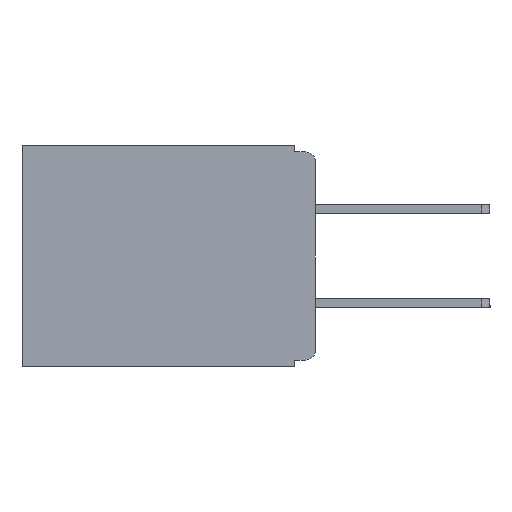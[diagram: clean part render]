
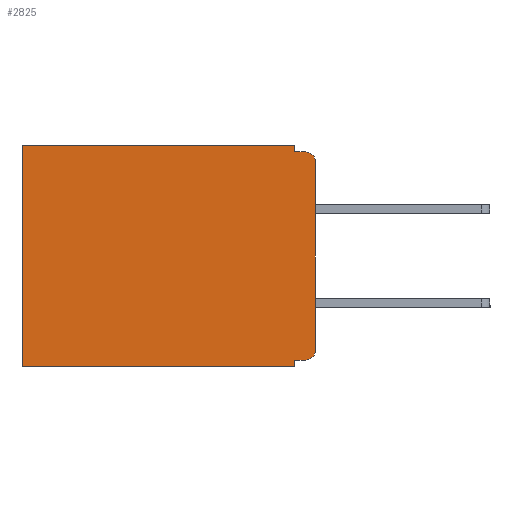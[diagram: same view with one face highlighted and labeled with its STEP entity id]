
A CAD part, left-side view. The second image highlights one B-rep face of the part: STEP entity #2825.
In plain terms, the highlighted planar face has unit normal (-1, 0, 0).
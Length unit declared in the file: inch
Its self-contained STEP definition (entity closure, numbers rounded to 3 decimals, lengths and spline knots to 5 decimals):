
#13 = ORIENTED_EDGE ( 'NONE', *, *, #7940, .T. ) ;
#251 = ORIENTED_EDGE ( 'NONE', *, *, #16608, .T. ) ;
#423 = EDGE_CURVE ( 'NONE', #15945, #10804, #10420, .T. ) ;
#532 = ORIENTED_EDGE ( 'NONE', *, *, #8888, .F. ) ;
#535 = DIRECTION ( 'NONE',  ( 0., 1., 0. ) ) ;
#1096 = ORIENTED_EDGE ( 'NONE', *, *, #5507, .F. ) ;
#1252 = ORIENTED_EDGE ( 'NONE', *, *, #423, .T. ) ;
#1308 = EDGE_CURVE ( 'NONE', #12455, #4254, #18576, .T. ) ;
#1642 = LINE ( 'NONE', #11935, #13203 ) ;
#1795 = CARTESIAN_POINT ( 'NONE',  ( 0.3, 0.031, 0. ) ) ;
#2652 = DIRECTION ( 'NONE',  ( -1., 0., 0. ) ) ;
#2656 = VERTEX_POINT ( 'NONE', #4014 ) ;
#2825 = ADVANCED_FACE ( 'NONE', ( #13002 ), #16851, .F. ) ;
#2857 = CARTESIAN_POINT ( 'NONE',  ( 0.3, 0., -0.33 ) ) ;
#2863 = DIRECTION ( 'NONE',  ( 0., 0., -1. ) ) ;
#3182 = EDGE_CURVE ( 'NONE', #6920, #4254, #11863, .T. ) ;
#3349 = VECTOR ( 'NONE', #5999, 39.37008 ) ;
#3707 = CARTESIAN_POINT ( 'NONE',  ( 0.3, 0.437, -0.33 ) ) ;
#4014 = CARTESIAN_POINT ( 'NONE',  ( 0.3, 0.031, -0.01 ) ) ;
#4216 = CIRCLE ( 'NONE', #11251, 0.015 ) ;
#4254 = VERTEX_POINT ( 'NONE', #3707 ) ;
#4491 = LINE ( 'NONE', #16780, #12026 ) ;
#5507 = EDGE_CURVE ( 'NONE', #2656, #15579, #18805, .T. ) ;
#5581 = ORIENTED_EDGE ( 'NONE', *, *, #7904, .F. ) ;
#5868 = ORIENTED_EDGE ( 'NONE', *, *, #1308, .F. ) ;
#5924 = ORIENTED_EDGE ( 'NONE', *, *, #3182, .T. ) ;
#5999 = DIRECTION ( 'NONE',  ( 0., 0., -1. ) ) ;
#6069 = VERTEX_POINT ( 'NONE', #14376 ) ;
#6560 = DIRECTION ( 'NONE',  ( 0., -1., 0. ) ) ;
#6920 = VERTEX_POINT ( 'NONE', #17033 ) ;
#7224 = CARTESIAN_POINT ( 'NONE',  ( 0.3, 0., -0.01 ) ) ;
#7368 = ORIENTED_EDGE ( 'NONE', *, *, #13841, .F. ) ;
#7381 = DIRECTION ( 'NONE',  ( 0., 0., -1. ) ) ;
#7577 = VECTOR ( 'NONE', #6560, 39.37008 ) ;
#7847 = ORIENTED_EDGE ( 'NONE', *, *, #17361, .F. ) ;
#7904 = EDGE_CURVE ( 'NONE', #6069, #12455, #16985, .T. ) ;
#7940 = EDGE_CURVE ( 'NONE', #9602, #15579, #4216, .T. ) ;
#7973 = CARTESIAN_POINT ( 'NONE',  ( 0.3, 0., -0.33 ) ) ;
#8722 = DIRECTION ( 'NONE',  ( 0., 1., 0. ) ) ;
#8888 = EDGE_CURVE ( 'NONE', #15779, #2656, #19001, .T. ) ;
#9524 = DIRECTION ( 'NONE',  ( 0., 1., 0. ) ) ;
#9602 = VERTEX_POINT ( 'NONE', #13423 ) ;
#10281 = AXIS2_PLACEMENT_3D ( 'NONE', #18841, #2652, #2863 ) ;
#10314 = DIRECTION ( 'NONE',  ( 0., 0., -1. ) ) ;
#10359 = VECTOR ( 'NONE', #7381, 39.37008 ) ;
#10362 = DIRECTION ( 'NONE',  ( -1., 0., 0. ) ) ;
#10381 = CARTESIAN_POINT ( 'NONE',  ( 0.3, 0.015, -0.025 ) ) ;
#10420 = CIRCLE ( 'NONE', #10281, 0.015 ) ;
#10777 = DIRECTION ( 'NONE',  ( 0., 0., -1. ) ) ;
#10804 = VERTEX_POINT ( 'NONE', #16427 ) ;
#10861 = CARTESIAN_POINT ( 'NONE',  ( 0.3, 0.031, -0.33 ) ) ;
#11251 = AXIS2_PLACEMENT_3D ( 'NONE', #10381, #10362, #10314 ) ;
#11353 = CARTESIAN_POINT ( 'NONE',  ( 0.3, 0.015, -0.32 ) ) ;
#11863 = LINE ( 'NONE', #16821, #3349 ) ;
#11935 = CARTESIAN_POINT ( 'NONE',  ( 0.3, 0., -0.33 ) ) ;
#12026 = VECTOR ( 'NONE', #9524, 39.37008 ) ;
#12348 = LINE ( 'NONE', #18947, #19133 ) ;
#12455 = VERTEX_POINT ( 'NONE', #17919 ) ;
#13002 = FACE_OUTER_BOUND ( 'NONE', #13007, .T. ) ;
#13007 = EDGE_LOOP ( 'NONE', ( #7847, #13, #1096, #532, #251, #5924, #5868, #5581, #7368, #1252 ) ) ;
#13203 = VECTOR ( 'NONE', #13376, 39.37008 ) ;
#13376 = DIRECTION ( 'NONE',  ( 0., 0., -1. ) ) ;
#13423 = CARTESIAN_POINT ( 'NONE',  ( 0.3, 0., -0.025 ) ) ;
#13841 = EDGE_CURVE ( 'NONE', #15945, #6069, #4491, .T. ) ;
#14198 = AXIS2_PLACEMENT_3D ( 'NONE', #7973, #18688, #17633 ) ;
#14232 = VECTOR ( 'NONE', #535, 39.37008 ) ;
#14376 = CARTESIAN_POINT ( 'NONE',  ( 0.3, 0.031, -0.32 ) ) ;
#15579 = VERTEX_POINT ( 'NONE', #16243 ) ;
#15779 = VERTEX_POINT ( 'NONE', #1795 ) ;
#15945 = VERTEX_POINT ( 'NONE', #11353 ) ;
#16066 = VECTOR ( 'NONE', #10777, 39.37008 ) ;
#16243 = CARTESIAN_POINT ( 'NONE',  ( 0.3, 0.015, -0.01 ) ) ;
#16427 = CARTESIAN_POINT ( 'NONE',  ( 0.3, 0., -0.305 ) ) ;
#16608 = EDGE_CURVE ( 'NONE', #15779, #6920, #12348, .T. ) ;
#16780 = CARTESIAN_POINT ( 'NONE',  ( 0.3, 0., -0.32 ) ) ;
#16821 = CARTESIAN_POINT ( 'NONE',  ( 0.3, 0.437, -0.33 ) ) ;
#16851 = PLANE ( 'NONE',  #14198 ) ;
#16985 = LINE ( 'NONE', #10861, #16066 ) ;
#17033 = CARTESIAN_POINT ( 'NONE',  ( 0.3, 0.437, 0. ) ) ;
#17361 = EDGE_CURVE ( 'NONE', #9602, #10804, #1642, .T. ) ;
#17567 = CARTESIAN_POINT ( 'NONE',  ( 0.3, 0.031, 0. ) ) ;
#17633 = DIRECTION ( 'NONE',  ( 0., 0., -1. ) ) ;
#17919 = CARTESIAN_POINT ( 'NONE',  ( 0.3, 0.031, -0.33 ) ) ;
#18576 = LINE ( 'NONE', #2857, #14232 ) ;
#18688 = DIRECTION ( 'NONE',  ( 1., 0., 0. ) ) ;
#18805 = LINE ( 'NONE', #7224, #7577 ) ;
#18841 = CARTESIAN_POINT ( 'NONE',  ( 0.3, 0.015, -0.305 ) ) ;
#18947 = CARTESIAN_POINT ( 'NONE',  ( 0.3, 0., 0. ) ) ;
#19001 = LINE ( 'NONE', #17567, #10359 ) ;
#19133 = VECTOR ( 'NONE', #8722, 39.37008 ) ;
